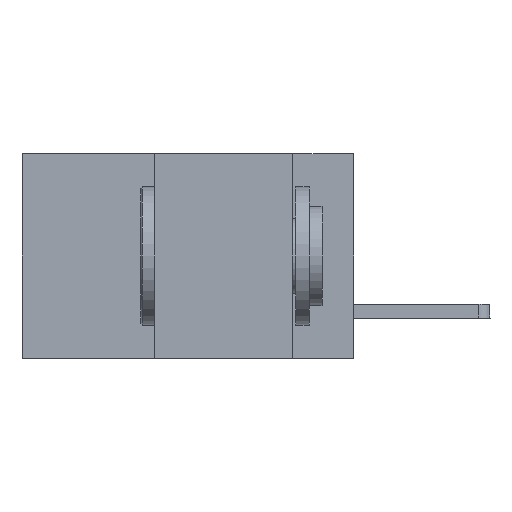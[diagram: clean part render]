
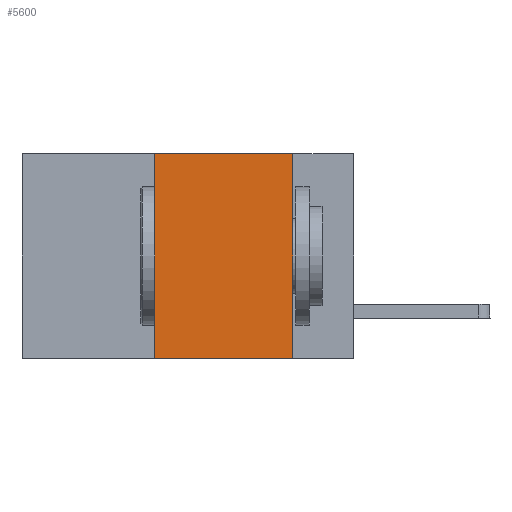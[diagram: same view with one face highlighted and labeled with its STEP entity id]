
A CAD part, left-side view. The second image highlights one B-rep face of the part: STEP entity #5600.
In plain terms, the highlighted planar face has unit normal (-1, 0, 0).
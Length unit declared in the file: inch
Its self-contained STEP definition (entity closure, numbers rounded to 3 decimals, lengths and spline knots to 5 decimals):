
#67 = CARTESIAN_POINT ( 'NONE',  ( 0., 0.6, -0.37 ) ) ;
#570 = LINE ( 'NONE', #10042, #6202 ) ;
#1009 = AXIS2_PLACEMENT_3D ( 'NONE', #2470, #3565, #3575 ) ;
#1536 = VECTOR ( 'NONE', #9448, 39.37008 ) ;
#1724 = EDGE_CURVE ( 'NONE', #9267, #4039, #7090, .T. ) ;
#1766 = ORIENTED_EDGE ( 'NONE', *, *, #9566, .T. ) ;
#1813 = CARTESIAN_POINT ( 'NONE',  ( 0., 0.11, 0. ) ) ;
#1925 = LINE ( 'NONE', #9451, #4274 ) ;
#2470 = CARTESIAN_POINT ( 'NONE',  ( 0., 0.6, 0. ) ) ;
#3065 = VECTOR ( 'NONE', #7956, 39.37008 ) ;
#3565 = DIRECTION ( 'NONE',  ( 1., 0., 0. ) ) ;
#3575 = DIRECTION ( 'NONE',  ( 0., 0., -1. ) ) ;
#3679 = PLANE ( 'NONE',  #1009 ) ;
#4039 = VERTEX_POINT ( 'NONE', #4682 ) ;
#4274 = VECTOR ( 'NONE', #9446, 39.37008 ) ;
#4682 = CARTESIAN_POINT ( 'NONE',  ( 0., 0.11, -0.37 ) ) ;
#5140 = ORIENTED_EDGE ( 'NONE', *, *, #6269, .F. ) ;
#5593 = ORIENTED_EDGE ( 'NONE', *, *, #1724, .F. ) ;
#5600 = ADVANCED_FACE ( 'NONE', ( #6407 ), #3679, .F. ) ;
#6202 = VECTOR ( 'NONE', #9841, 39.37008 ) ;
#6269 = EDGE_CURVE ( 'NONE', #10517, #9267, #1925, .T. ) ;
#6407 = FACE_OUTER_BOUND ( 'NONE', #12010, .T. ) ;
#6462 = CARTESIAN_POINT ( 'NONE',  ( 0., 0.36, 0. ) ) ;
#7090 = LINE ( 'NONE', #1813, #1536 ) ;
#7450 = CARTESIAN_POINT ( 'NONE',  ( 0., 0.11, 0. ) ) ;
#7610 = EDGE_CURVE ( 'NONE', #8418, #10517, #570, .T. ) ;
#7956 = DIRECTION ( 'NONE',  ( 0., -1., 0. ) ) ;
#8027 = CARTESIAN_POINT ( 'NONE',  ( 0., 0.36, -0.37 ) ) ;
#8196 = LINE ( 'NONE', #67, #3065 ) ;
#8349 = ORIENTED_EDGE ( 'NONE', *, *, #7610, .F. ) ;
#8418 = VERTEX_POINT ( 'NONE', #8027 ) ;
#9267 = VERTEX_POINT ( 'NONE', #7450 ) ;
#9446 = DIRECTION ( 'NONE',  ( 0., -1., 0. ) ) ;
#9448 = DIRECTION ( 'NONE',  ( 0., 0., -1. ) ) ;
#9451 = CARTESIAN_POINT ( 'NONE',  ( 0., 0.6, 0. ) ) ;
#9566 = EDGE_CURVE ( 'NONE', #8418, #4039, #8196, .T. ) ;
#9841 = DIRECTION ( 'NONE',  ( 0., 0., 1. ) ) ;
#10042 = CARTESIAN_POINT ( 'NONE',  ( 0., 0.36, 0. ) ) ;
#10517 = VERTEX_POINT ( 'NONE', #6462 ) ;
#12010 = EDGE_LOOP ( 'NONE', ( #5593, #5140, #8349, #1766 ) ) ;
